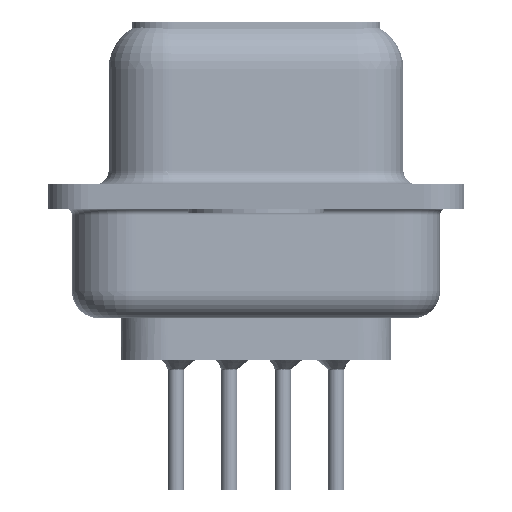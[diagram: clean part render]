
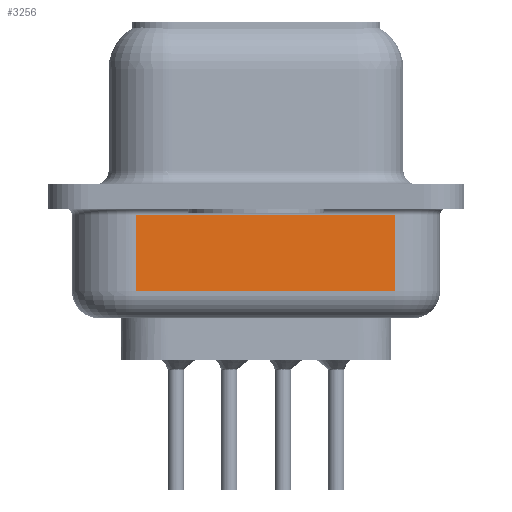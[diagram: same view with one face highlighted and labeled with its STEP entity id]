
A CAD part, left-side view. The second image highlights one B-rep face of the part: STEP entity #3256.
In plain terms, the highlighted planar face has unit normal (-0.985, -0.174, 0).
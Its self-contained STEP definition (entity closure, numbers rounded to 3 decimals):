
#1635 = DIRECTION ( 'NONE',  ( 0., 0., 1. ) ) ;
#3241 = VERTEX_POINT ( 'NONE', #46352 ) ;
#3256 = ADVANCED_FACE ( 'NONE', ( #50585 ), #20240, .F. ) ;
#5629 = LINE ( 'NONE', #31744, #12473 ) ;
#5860 = DIRECTION ( 'NONE',  ( 0.174, -0.985, 0. ) ) ;
#6643 = DIRECTION ( 'NONE',  ( 0., 0., 1. ) ) ;
#6930 = LINE ( 'NONE', #20013, #11926 ) ;
#9333 = ORIENTED_EDGE ( 'NONE', *, *, #38969, .T. ) ;
#11358 = ORIENTED_EDGE ( 'NONE', *, *, #55551, .F. ) ;
#11428 = CARTESIAN_POINT ( 'NONE',  ( 3.035, 4.453, -0.7 ) ) ;
#11926 = VECTOR ( 'NONE', #6643, 1000. ) ;
#12473 = VECTOR ( 'NONE', #1635, 1000. ) ;
#12681 = EDGE_LOOP ( 'NONE', ( #11358, #31921, #21275, #9333 ) ) ;
#14945 = CARTESIAN_POINT ( 'NONE',  ( 3.035, 4.453, -3.5 ) ) ;
#15154 = LINE ( 'NONE', #39652, #39521 ) ;
#15937 = VECTOR ( 'NONE', #5860, 1000. ) ;
#20013 = CARTESIAN_POINT ( 'NONE',  ( 3.035, 4.453, -4.5 ) ) ;
#20240 = PLANE ( 'NONE',  #54554 ) ;
#21275 = ORIENTED_EDGE ( 'NONE', *, *, #50339, .T. ) ;
#24686 = EDGE_CURVE ( 'NONE', #3241, #35796, #27446, .T. ) ;
#27446 = LINE ( 'NONE', #14945, #15937 ) ;
#31744 = CARTESIAN_POINT ( 'NONE',  ( 4.728, -5.147, -4.5 ) ) ;
#31921 = ORIENTED_EDGE ( 'NONE', *, *, #24686, .T. ) ;
#32463 = DIRECTION ( 'NONE',  ( -0.174, 0.985, 0. ) ) ;
#32979 = VERTEX_POINT ( 'NONE', #42351 ) ;
#35796 = VERTEX_POINT ( 'NONE', #55252 ) ;
#38969 = EDGE_CURVE ( 'NONE', #32979, #47831, #15154, .T. ) ;
#39521 = VECTOR ( 'NONE', #32463, 1000. ) ;
#39652 = CARTESIAN_POINT ( 'NONE',  ( 3.035, 4.453, -0.7 ) ) ;
#42351 = CARTESIAN_POINT ( 'NONE',  ( 4.728, -5.147, -0.7 ) ) ;
#46352 = CARTESIAN_POINT ( 'NONE',  ( 3.035, 4.453, -3.5 ) ) ;
#47193 = DIRECTION ( 'NONE',  ( 0.985, 0.174, 0. ) ) ;
#47831 = VERTEX_POINT ( 'NONE', #11428 ) ;
#50339 = EDGE_CURVE ( 'NONE', #35796, #32979, #5629, .T. ) ;
#50585 = FACE_OUTER_BOUND ( 'NONE', #12681, .T. ) ;
#51985 = DIRECTION ( 'NONE',  ( -0.174, 0.985, 0. ) ) ;
#54554 = AXIS2_PLACEMENT_3D ( 'NONE', #54829, #47193, #51985 ) ;
#54829 = CARTESIAN_POINT ( 'NONE',  ( 3.035, 4.453, -4.5 ) ) ;
#55252 = CARTESIAN_POINT ( 'NONE',  ( 4.728, -5.147, -3.5 ) ) ;
#55551 = EDGE_CURVE ( 'NONE', #3241, #47831, #6930, .T. ) ;
